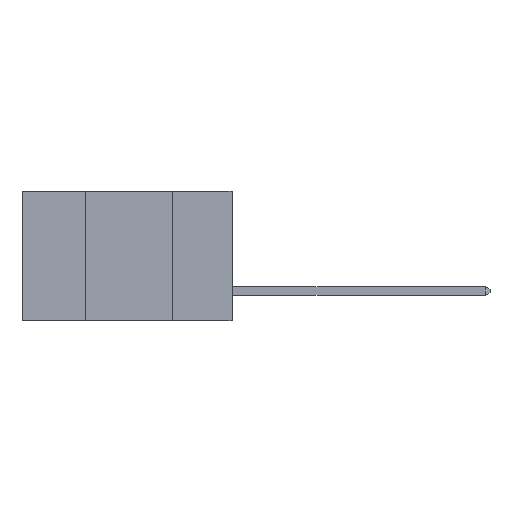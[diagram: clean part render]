
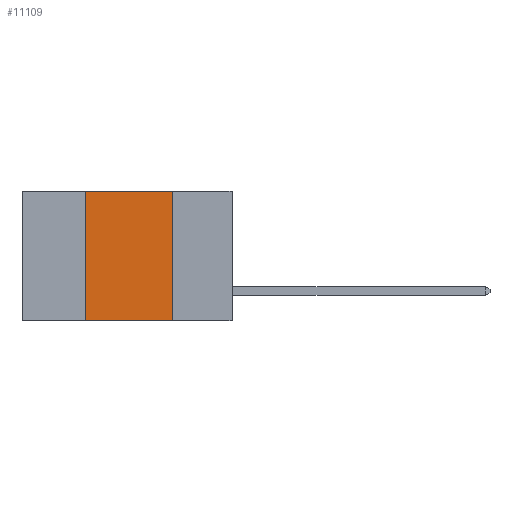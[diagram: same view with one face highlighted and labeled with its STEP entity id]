
A CAD part, left-side view. The second image highlights one B-rep face of the part: STEP entity #11109.
In plain terms, the highlighted planar face has unit normal (-1, 0, 0).
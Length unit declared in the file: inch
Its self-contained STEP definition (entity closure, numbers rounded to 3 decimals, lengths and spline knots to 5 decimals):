
#915 = VERTEX_POINT ( 'NONE', #5195 ) ;
#1016 = CARTESIAN_POINT ( 'NONE',  ( 0., 0.6, 0. ) ) ;
#1022 = CARTESIAN_POINT ( 'NONE',  ( 0., 0.42, 0. ) ) ;
#1320 = CARTESIAN_POINT ( 'NONE',  ( 0., 0.42, 0. ) ) ;
#1550 = EDGE_CURVE ( 'NONE', #14822, #915, #9301, .T. ) ;
#1606 = LINE ( 'NONE', #1016, #8934 ) ;
#1795 = EDGE_LOOP ( 'NONE', ( #19933, #2030, #6531, #9350 ) ) ;
#2030 = ORIENTED_EDGE ( 'NONE', *, *, #16412, .F. ) ;
#2235 = VECTOR ( 'NONE', #2981, 39.37008 ) ;
#2981 = DIRECTION ( 'NONE',  ( 0., 0., 1. ) ) ;
#3021 = VECTOR ( 'NONE', #13688, 39.37008 ) ;
#3423 = PLANE ( 'NONE',  #6648 ) ;
#4100 = VERTEX_POINT ( 'NONE', #1022 ) ;
#5114 = CARTESIAN_POINT ( 'NONE',  ( 0., 0.6, 0. ) ) ;
#5195 = CARTESIAN_POINT ( 'NONE',  ( 0., 0.17, -0.37 ) ) ;
#6390 = CARTESIAN_POINT ( 'NONE',  ( 0., 0.6, -0.37 ) ) ;
#6531 = ORIENTED_EDGE ( 'NONE', *, *, #13615, .F. ) ;
#6648 = AXIS2_PLACEMENT_3D ( 'NONE', #5114, #17805, #8488 ) ;
#8488 = DIRECTION ( 'NONE',  ( 0., 0., -1. ) ) ;
#8520 = LINE ( 'NONE', #12142, #3021 ) ;
#8934 = VECTOR ( 'NONE', #10973, 39.37008 ) ;
#9301 = LINE ( 'NONE', #6390, #10294 ) ;
#9350 = ORIENTED_EDGE ( 'NONE', *, *, #1550, .T. ) ;
#10294 = VECTOR ( 'NONE', #16604, 39.37008 ) ;
#10973 = DIRECTION ( 'NONE',  ( 0., -1., 0. ) ) ;
#11057 = LINE ( 'NONE', #1320, #2235 ) ;
#11109 = ADVANCED_FACE ( 'NONE', ( #14197 ), #3423, .F. ) ;
#12142 = CARTESIAN_POINT ( 'NONE',  ( 0., 0.17, 0. ) ) ;
#13615 = EDGE_CURVE ( 'NONE', #14822, #4100, #11057, .T. ) ;
#13688 = DIRECTION ( 'NONE',  ( 0., 0., -1. ) ) ;
#14197 = FACE_OUTER_BOUND ( 'NONE', #1795, .T. ) ;
#14822 = VERTEX_POINT ( 'NONE', #20423 ) ;
#16412 = EDGE_CURVE ( 'NONE', #4100, #16525, #1606, .T. ) ;
#16525 = VERTEX_POINT ( 'NONE', #20338 ) ;
#16604 = DIRECTION ( 'NONE',  ( 0., -1., 0. ) ) ;
#17805 = DIRECTION ( 'NONE',  ( 1., 0., 0. ) ) ;
#18585 = EDGE_CURVE ( 'NONE', #16525, #915, #8520, .T. ) ;
#19933 = ORIENTED_EDGE ( 'NONE', *, *, #18585, .F. ) ;
#20338 = CARTESIAN_POINT ( 'NONE',  ( 0., 0.17, 0. ) ) ;
#20423 = CARTESIAN_POINT ( 'NONE',  ( 0., 0.42, -0.37 ) ) ;
